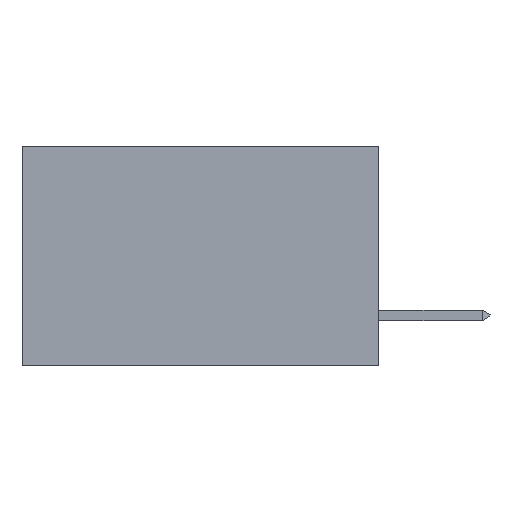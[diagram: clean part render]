
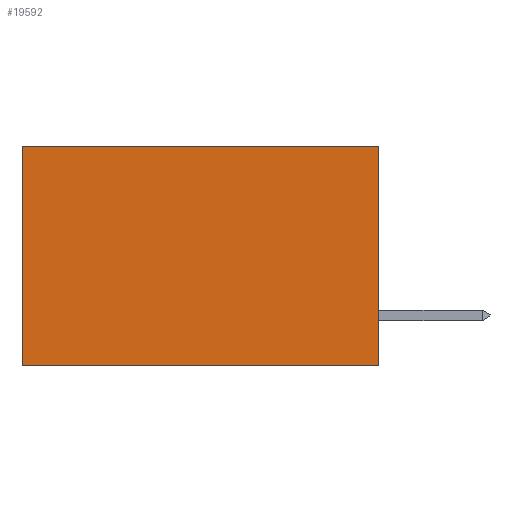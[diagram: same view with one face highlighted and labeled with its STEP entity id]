
A CAD part, left-side view. The second image highlights one B-rep face of the part: STEP entity #19592.
In plain terms, the highlighted planar face has unit normal (-1, 0, 0).
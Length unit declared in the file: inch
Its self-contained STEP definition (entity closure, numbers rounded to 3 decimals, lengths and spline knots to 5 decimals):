
#1555 = VECTOR ( 'NONE', #13920, 39.37008 ) ;
#2881 = ORIENTED_EDGE ( 'NONE', *, *, #5825, .F. ) ;
#3431 = FACE_OUTER_BOUND ( 'NONE', #18057, .T. ) ;
#3512 = CARTESIAN_POINT ( 'NONE',  ( 0.2615, 0.6, 0. ) ) ;
#3836 = VERTEX_POINT ( 'NONE', #21121 ) ;
#4083 = DIRECTION ( 'NONE',  ( 0., 1., 0. ) ) ;
#4748 = VERTEX_POINT ( 'NONE', #4897 ) ;
#4749 = CARTESIAN_POINT ( 'NONE',  ( 0.2615, 0., -0.37 ) ) ;
#4897 = CARTESIAN_POINT ( 'NONE',  ( 0.2615, 0., -0.37 ) ) ;
#5223 = VECTOR ( 'NONE', #22135, 39.37008 ) ;
#5822 = VECTOR ( 'NONE', #21352, 39.37008 ) ;
#5825 = EDGE_CURVE ( 'NONE', #4748, #3836, #6880, .T. ) ;
#6767 = CARTESIAN_POINT ( 'NONE',  ( 0.2615, 0., -0.37 ) ) ;
#6880 = LINE ( 'NONE', #6767, #5822 ) ;
#7783 = CARTESIAN_POINT ( 'NONE',  ( 0.2615, 0., 0. ) ) ;
#8136 = LINE ( 'NONE', #7783, #9080 ) ;
#9080 = VECTOR ( 'NONE', #4083, 39.37008 ) ;
#10853 = ORIENTED_EDGE ( 'NONE', *, *, #13281, .F. ) ;
#13145 = AXIS2_PLACEMENT_3D ( 'NONE', #4749, #22079, #20405 ) ;
#13281 = EDGE_CURVE ( 'NONE', #17670, #4748, #23001, .T. ) ;
#13920 = DIRECTION ( 'NONE',  ( 0., 0., -1. ) ) ;
#15064 = CARTESIAN_POINT ( 'NONE',  ( 0.2615, 0., 0. ) ) ;
#16423 = ORIENTED_EDGE ( 'NONE', *, *, #23229, .T. ) ;
#17670 = VERTEX_POINT ( 'NONE', #15064 ) ;
#18057 = EDGE_LOOP ( 'NONE', ( #16423, #2881, #10853, #21100 ) ) ;
#19592 = ADVANCED_FACE ( 'NONE', ( #3431 ), #21141, .F. ) ;
#20226 = LINE ( 'NONE', #23458, #5223 ) ;
#20405 = DIRECTION ( 'NONE',  ( 0., 0., -1. ) ) ;
#21100 = ORIENTED_EDGE ( 'NONE', *, *, #23340, .T. ) ;
#21121 = CARTESIAN_POINT ( 'NONE',  ( 0.2615, 0.6, -0.37 ) ) ;
#21141 = PLANE ( 'NONE',  #13145 ) ;
#21340 = CARTESIAN_POINT ( 'NONE',  ( 0.2615, 0., -0.37 ) ) ;
#21352 = DIRECTION ( 'NONE',  ( 0., 1., 0. ) ) ;
#21519 = VERTEX_POINT ( 'NONE', #3512 ) ;
#22079 = DIRECTION ( 'NONE',  ( 1., 0., 0. ) ) ;
#22135 = DIRECTION ( 'NONE',  ( 0., 0., -1. ) ) ;
#23001 = LINE ( 'NONE', #21340, #1555 ) ;
#23229 = EDGE_CURVE ( 'NONE', #21519, #3836, #20226, .T. ) ;
#23340 = EDGE_CURVE ( 'NONE', #17670, #21519, #8136, .T. ) ;
#23458 = CARTESIAN_POINT ( 'NONE',  ( 0.2615, 0.6, -0.37 ) ) ;
